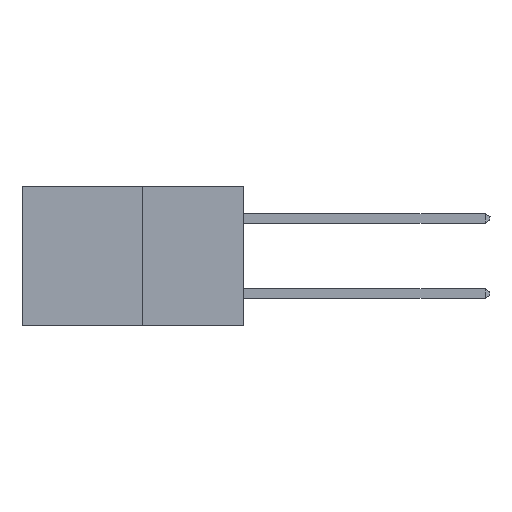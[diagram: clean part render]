
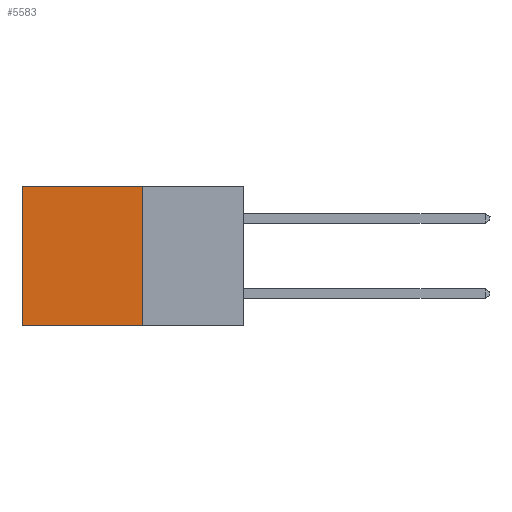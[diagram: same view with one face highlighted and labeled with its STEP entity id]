
A CAD part, left-side view. The second image highlights one B-rep face of the part: STEP entity #5583.
In plain terms, the highlighted planar face has unit normal (-1, 0, 0).
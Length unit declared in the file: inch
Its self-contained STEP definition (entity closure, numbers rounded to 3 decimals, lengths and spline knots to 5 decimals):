
#414 = LINE ( 'NONE', #4854, #11339 ) ;
#846 = CARTESIAN_POINT ( 'NONE',  ( 0.277, 0.59, -0.37 ) ) ;
#1755 = VERTEX_POINT ( 'NONE', #13666 ) ;
#2292 = CARTESIAN_POINT ( 'NONE',  ( 0.277, 0.59, 0. ) ) ;
#2471 = DIRECTION ( 'NONE',  ( 0., 0., -1. ) ) ;
#2496 = VECTOR ( 'NONE', #11648, 39.37008 ) ;
#2819 = CARTESIAN_POINT ( 'NONE',  ( 0.277, 0.27, 0. ) ) ;
#2827 = ORIENTED_EDGE ( 'NONE', *, *, #12605, .F. ) ;
#4582 = CARTESIAN_POINT ( 'NONE',  ( 0.277, 0.59, -0.37 ) ) ;
#4624 = EDGE_CURVE ( 'NONE', #15435, #11209, #13791, .T. ) ;
#4854 = CARTESIAN_POINT ( 'NONE',  ( 0.277, 0.27, -0.37 ) ) ;
#5583 = ADVANCED_FACE ( 'NONE', ( #12849 ), #12291, .F. ) ;
#7268 = EDGE_LOOP ( 'NONE', ( #16528, #16969, #2827, #10795 ) ) ;
#8124 = CARTESIAN_POINT ( 'NONE',  ( 0.277, 0.27, -0.37 ) ) ;
#9546 = DIRECTION ( 'NONE',  ( 0., 0., -1. ) ) ;
#9890 = EDGE_CURVE ( 'NONE', #13381, #15435, #11402, .T. ) ;
#10795 = ORIENTED_EDGE ( 'NONE', *, *, #9890, .T. ) ;
#10927 = LINE ( 'NONE', #18027, #17988 ) ;
#10944 = VECTOR ( 'NONE', #15954, 39.37008 ) ;
#11209 = VERTEX_POINT ( 'NONE', #846 ) ;
#11339 = VECTOR ( 'NONE', #11976, 39.37008 ) ;
#11402 = LINE ( 'NONE', #15892, #10944 ) ;
#11648 = DIRECTION ( 'NONE',  ( 0., 0., -1. ) ) ;
#11976 = DIRECTION ( 'NONE',  ( 0., 1., 0. ) ) ;
#12291 = PLANE ( 'NONE',  #17079 ) ;
#12605 = EDGE_CURVE ( 'NONE', #13381, #1755, #10927, .T. ) ;
#12849 = FACE_OUTER_BOUND ( 'NONE', #7268, .T. ) ;
#13381 = VERTEX_POINT ( 'NONE', #2819 ) ;
#13666 = CARTESIAN_POINT ( 'NONE',  ( 0.277, 0.27, -0.37 ) ) ;
#13791 = LINE ( 'NONE', #4582, #2496 ) ;
#14651 = EDGE_CURVE ( 'NONE', #1755, #11209, #414, .T. ) ;
#15435 = VERTEX_POINT ( 'NONE', #2292 ) ;
#15892 = CARTESIAN_POINT ( 'NONE',  ( 0.277, 0.27, 0. ) ) ;
#15954 = DIRECTION ( 'NONE',  ( 0., 1., 0. ) ) ;
#16528 = ORIENTED_EDGE ( 'NONE', *, *, #4624, .T. ) ;
#16969 = ORIENTED_EDGE ( 'NONE', *, *, #14651, .F. ) ;
#17079 = AXIS2_PLACEMENT_3D ( 'NONE', #8124, #18013, #9546 ) ;
#17988 = VECTOR ( 'NONE', #2471, 39.37008 ) ;
#18013 = DIRECTION ( 'NONE',  ( 1., 0., 0. ) ) ;
#18027 = CARTESIAN_POINT ( 'NONE',  ( 0.277, 0.27, -0.37 ) ) ;
